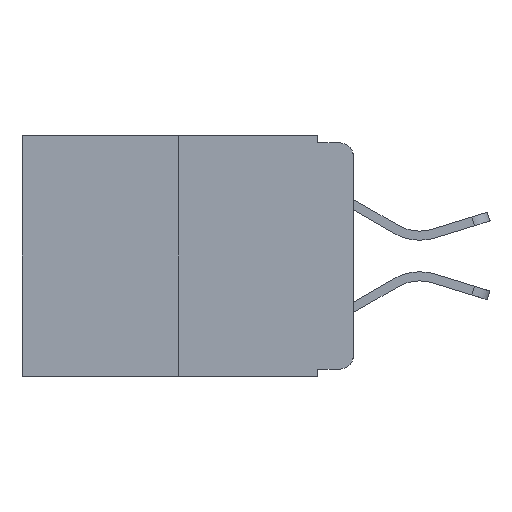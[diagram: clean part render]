
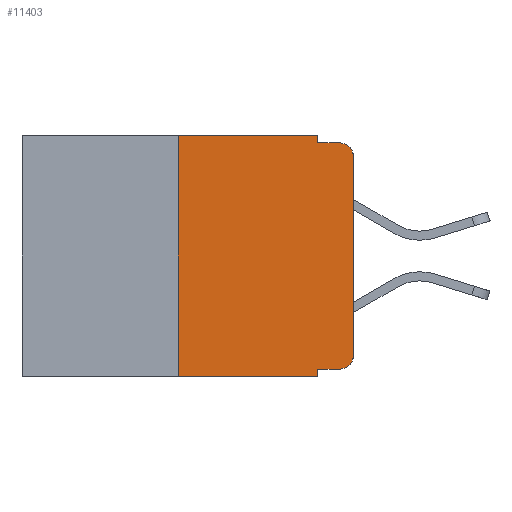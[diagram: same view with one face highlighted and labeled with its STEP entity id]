
A CAD part, left-side view. The second image highlights one B-rep face of the part: STEP entity #11403.
In plain terms, the highlighted planar face has unit normal (-1, 0, 0).
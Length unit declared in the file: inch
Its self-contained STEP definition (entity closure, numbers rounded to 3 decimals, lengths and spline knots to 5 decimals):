
#331 = VECTOR ( 'NONE', #14660, 39.37008 ) ;
#770 = VERTEX_POINT ( 'NONE', #9122 ) ;
#1113 = CARTESIAN_POINT ( 'NONE',  ( 0., 0.051, 0. ) ) ;
#1498 = VECTOR ( 'NONE', #6816, 39.37008 ) ;
#1595 = VERTEX_POINT ( 'NONE', #7242 ) ;
#1786 = LINE ( 'NONE', #17436, #16557 ) ;
#2104 = EDGE_CURVE ( 'NONE', #18836, #4573, #17622, .T. ) ;
#2239 = DIRECTION ( 'NONE',  ( 0., -1., 0. ) ) ;
#2320 = DIRECTION ( 'NONE',  ( 0., 0., 1. ) ) ;
#2800 = CARTESIAN_POINT ( 'NONE',  ( 0., 0.473, -0.343 ) ) ;
#2804 = AXIS2_PLACEMENT_3D ( 'NONE', #12143, #16755, #3186 ) ;
#2845 = DIRECTION ( 'NONE',  ( 0., 0., -1. ) ) ;
#3186 = DIRECTION ( 'NONE',  ( 0., 0., -1. ) ) ;
#3251 = CARTESIAN_POINT ( 'NONE',  ( 0., 0.051, -0.01 ) ) ;
#3333 = VECTOR ( 'NONE', #2239, 39.37008 ) ;
#3449 = VERTEX_POINT ( 'NONE', #16507 ) ;
#3693 = DIRECTION ( 'NONE',  ( 0., 0., -1. ) ) ;
#4079 = AXIS2_PLACEMENT_3D ( 'NONE', #19400, #19337, #2845 ) ;
#4139 = VERTEX_POINT ( 'NONE', #3251 ) ;
#4417 = VERTEX_POINT ( 'NONE', #1113 ) ;
#4477 = LINE ( 'NONE', #18775, #3333 ) ;
#4573 = VERTEX_POINT ( 'NONE', #5987 ) ;
#4892 = EDGE_CURVE ( 'NONE', #16149, #1595, #11133, .T. ) ;
#5092 = EDGE_CURVE ( 'NONE', #4417, #4139, #12040, .T. ) ;
#5330 = CARTESIAN_POINT ( 'NONE',  ( 0., 0., -0.313 ) ) ;
#5493 = PLANE ( 'NONE',  #4079 ) ;
#5517 = DIRECTION ( 'NONE',  ( 0., -1., 0. ) ) ;
#5822 = LINE ( 'NONE', #2800, #8596 ) ;
#5829 = AXIS2_PLACEMENT_3D ( 'NONE', #14095, #12657, #3693 ) ;
#5840 = CIRCLE ( 'NONE', #2804, 0.02 ) ;
#5987 = CARTESIAN_POINT ( 'NONE',  ( 0., 0.25, 0. ) ) ;
#6483 = CARTESIAN_POINT ( 'NONE',  ( 0., 0.051, -0.333 ) ) ;
#6662 = ORIENTED_EDGE ( 'NONE', *, *, #13809, .T. ) ;
#6816 = DIRECTION ( 'NONE',  ( 0., 0., -1. ) ) ;
#7232 = VERTEX_POINT ( 'NONE', #5330 ) ;
#7242 = CARTESIAN_POINT ( 'NONE',  ( 0., 0.051, -0.343 ) ) ;
#7267 = VECTOR ( 'NONE', #10037, 39.37008 ) ;
#7796 = EDGE_CURVE ( 'NONE', #4139, #18091, #16170, .T. ) ;
#8094 = EDGE_CURVE ( 'NONE', #770, #7232, #5840, .T. ) ;
#8208 = EDGE_CURVE ( 'NONE', #3449, #18091, #9107, .T. ) ;
#8566 = ORIENTED_EDGE ( 'NONE', *, *, #8208, .T. ) ;
#8596 = VECTOR ( 'NONE', #13138, 39.37008 ) ;
#8744 = EDGE_CURVE ( 'NONE', #18836, #1595, #5822, .T. ) ;
#9006 = CARTESIAN_POINT ( 'NONE',  ( 0., 0.25, -0.343 ) ) ;
#9107 = CIRCLE ( 'NONE', #5829, 0.02 ) ;
#9122 = CARTESIAN_POINT ( 'NONE',  ( 0., 0.02, -0.333 ) ) ;
#9279 = ORIENTED_EDGE ( 'NONE', *, *, #8094, .T. ) ;
#9744 = CARTESIAN_POINT ( 'NONE',  ( 0., 0.051, 0. ) ) ;
#10037 = DIRECTION ( 'NONE',  ( 0., -1., 0. ) ) ;
#10104 = VECTOR ( 'NONE', #2320, 39.37008 ) ;
#10159 = VECTOR ( 'NONE', #15453, 39.37008 ) ;
#10995 = ORIENTED_EDGE ( 'NONE', *, *, #2104, .F. ) ;
#11133 = LINE ( 'NONE', #14132, #10159 ) ;
#11403 = ADVANCED_FACE ( 'NONE', ( #15913 ), #5493, .F. ) ;
#11496 = EDGE_LOOP ( 'NONE', ( #6662, #8566, #16021, #12976, #15108, #10995, #17474, #17160, #13080, #9279 ) ) ;
#12040 = LINE ( 'NONE', #9744, #1498 ) ;
#12143 = CARTESIAN_POINT ( 'NONE',  ( 0., 0.02, -0.313 ) ) ;
#12657 = DIRECTION ( 'NONE',  ( -1., 0., 0. ) ) ;
#12976 = ORIENTED_EDGE ( 'NONE', *, *, #5092, .F. ) ;
#13080 = ORIENTED_EDGE ( 'NONE', *, *, #13854, .T. ) ;
#13138 = DIRECTION ( 'NONE',  ( 0., -1., 0. ) ) ;
#13809 = EDGE_CURVE ( 'NONE', #7232, #3449, #16319, .T. ) ;
#13854 = EDGE_CURVE ( 'NONE', #16149, #770, #1786, .T. ) ;
#14095 = CARTESIAN_POINT ( 'NONE',  ( 0., 0.02, -0.03 ) ) ;
#14132 = CARTESIAN_POINT ( 'NONE',  ( 0., 0.051, 0. ) ) ;
#14660 = DIRECTION ( 'NONE',  ( 0., 0., 1. ) ) ;
#15108 = ORIENTED_EDGE ( 'NONE', *, *, #18499, .F. ) ;
#15453 = DIRECTION ( 'NONE',  ( 0., 0., -1. ) ) ;
#15913 = FACE_OUTER_BOUND ( 'NONE', #11496, .T. ) ;
#15934 = CARTESIAN_POINT ( 'NONE',  ( 0., 0.25, 0. ) ) ;
#16021 = ORIENTED_EDGE ( 'NONE', *, *, #7796, .F. ) ;
#16149 = VERTEX_POINT ( 'NONE', #6483 ) ;
#16170 = LINE ( 'NONE', #19147, #7267 ) ;
#16319 = LINE ( 'NONE', #17496, #331 ) ;
#16507 = CARTESIAN_POINT ( 'NONE',  ( 0., 0., -0.03 ) ) ;
#16557 = VECTOR ( 'NONE', #5517, 39.37008 ) ;
#16755 = DIRECTION ( 'NONE',  ( -1., 0., 0. ) ) ;
#17160 = ORIENTED_EDGE ( 'NONE', *, *, #4892, .F. ) ;
#17436 = CARTESIAN_POINT ( 'NONE',  ( 0., 0.051, -0.333 ) ) ;
#17474 = ORIENTED_EDGE ( 'NONE', *, *, #8744, .T. ) ;
#17496 = CARTESIAN_POINT ( 'NONE',  ( 0., 0., 0. ) ) ;
#17622 = LINE ( 'NONE', #15934, #10104 ) ;
#17894 = CARTESIAN_POINT ( 'NONE',  ( 0., 0.02, -0.01 ) ) ;
#18091 = VERTEX_POINT ( 'NONE', #17894 ) ;
#18499 = EDGE_CURVE ( 'NONE', #4573, #4417, #4477, .T. ) ;
#18775 = CARTESIAN_POINT ( 'NONE',  ( 0., 0.473, 0. ) ) ;
#18836 = VERTEX_POINT ( 'NONE', #9006 ) ;
#19147 = CARTESIAN_POINT ( 'NONE',  ( 0., 0.051, -0.01 ) ) ;
#19337 = DIRECTION ( 'NONE',  ( 1., 0., 0. ) ) ;
#19400 = CARTESIAN_POINT ( 'NONE',  ( 0., 0.473, 0. ) ) ;
